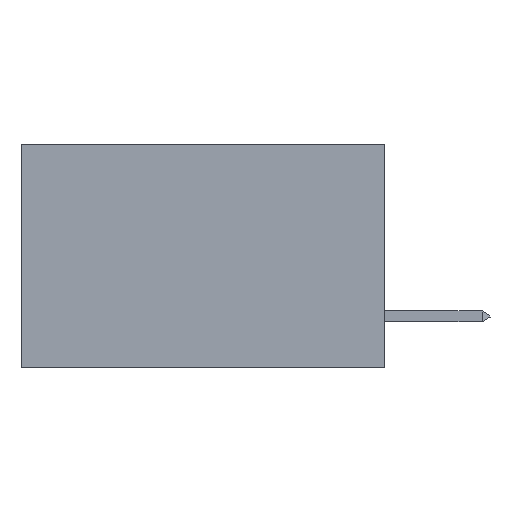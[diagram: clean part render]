
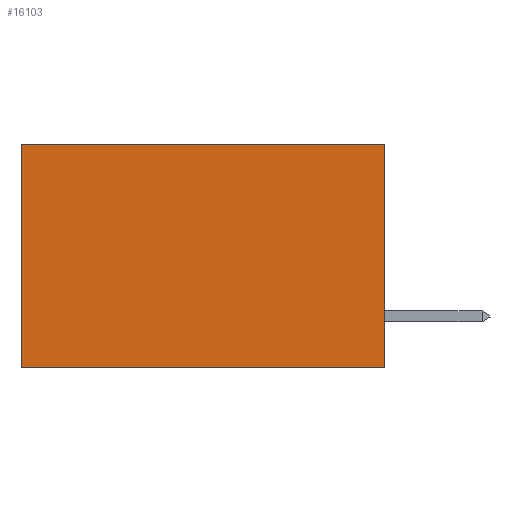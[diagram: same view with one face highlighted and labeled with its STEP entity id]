
A CAD part, left-side view. The second image highlights one B-rep face of the part: STEP entity #16103.
In plain terms, the highlighted planar face has unit normal (-1, 0, 0).
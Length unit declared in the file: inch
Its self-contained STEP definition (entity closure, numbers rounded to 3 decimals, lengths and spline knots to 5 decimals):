
#881 = LINE ( 'NONE', #18481, #15716 ) ;
#1019 = CARTESIAN_POINT ( 'NONE',  ( 0.2875, 0.6, 0. ) ) ;
#1499 = DIRECTION ( 'NONE',  ( 1., 0., 0. ) ) ;
#3139 = EDGE_CURVE ( 'NONE', #24660, #46888, #36506, .T. ) ;
#5640 = CARTESIAN_POINT ( 'NONE',  ( 0.2875, 0., 0. ) ) ;
#6391 = CARTESIAN_POINT ( 'NONE',  ( 0.2875, 0.6, -0.37 ) ) ;
#10272 = VECTOR ( 'NONE', #20162, 39.37008 ) ;
#12434 = DIRECTION ( 'NONE',  ( 0., 0., -1. ) ) ;
#12813 = ORIENTED_EDGE ( 'NONE', *, *, #15578, .T. ) ;
#15257 = CARTESIAN_POINT ( 'NONE',  ( 0.2875, 0., 0. ) ) ;
#15578 = EDGE_CURVE ( 'NONE', #41574, #24660, #20748, .T. ) ;
#15716 = VECTOR ( 'NONE', #28354, 39.37008 ) ;
#16103 = ADVANCED_FACE ( 'NONE', ( #20079 ), #25756, .F. ) ;
#17558 = ORIENTED_EDGE ( 'NONE', *, *, #18643, .F. ) ;
#18376 = EDGE_LOOP ( 'NONE', ( #21313, #17558, #28267, #12813 ) ) ;
#18481 = CARTESIAN_POINT ( 'NONE',  ( 0.2875, 0., -0.37 ) ) ;
#18643 = EDGE_CURVE ( 'NONE', #19764, #46888, #881, .T. ) ;
#19764 = VERTEX_POINT ( 'NONE', #24697 ) ;
#20079 = FACE_OUTER_BOUND ( 'NONE', #18376, .T. ) ;
#20162 = DIRECTION ( 'NONE',  ( 0., 1., 0. ) ) ;
#20748 = LINE ( 'NONE', #5640, #10272 ) ;
#21313 = ORIENTED_EDGE ( 'NONE', *, *, #3139, .T. ) ;
#22531 = EDGE_CURVE ( 'NONE', #41574, #19764, #46314, .T. ) ;
#24525 = DIRECTION ( 'NONE',  ( 0., 0., -1. ) ) ;
#24660 = VERTEX_POINT ( 'NONE', #1019 ) ;
#24697 = CARTESIAN_POINT ( 'NONE',  ( 0.2875, 0., -0.37 ) ) ;
#25756 = PLANE ( 'NONE',  #38266 ) ;
#26475 = CARTESIAN_POINT ( 'NONE',  ( 0.2875, 0.6, 0. ) ) ;
#28267 = ORIENTED_EDGE ( 'NONE', *, *, #22531, .F. ) ;
#28354 = DIRECTION ( 'NONE',  ( 0., 1., 0. ) ) ;
#31080 = VECTOR ( 'NONE', #47416, 39.37008 ) ;
#36506 = LINE ( 'NONE', #26475, #47590 ) ;
#37107 = CARTESIAN_POINT ( 'NONE',  ( 0.2875, 0., 0. ) ) ;
#38266 = AXIS2_PLACEMENT_3D ( 'NONE', #15257, #1499, #24525 ) ;
#39720 = CARTESIAN_POINT ( 'NONE',  ( 0.2875, 0., 0. ) ) ;
#41574 = VERTEX_POINT ( 'NONE', #37107 ) ;
#46314 = LINE ( 'NONE', #39720, #31080 ) ;
#46888 = VERTEX_POINT ( 'NONE', #6391 ) ;
#47416 = DIRECTION ( 'NONE',  ( 0., 0., -1. ) ) ;
#47590 = VECTOR ( 'NONE', #12434, 39.37008 ) ;
